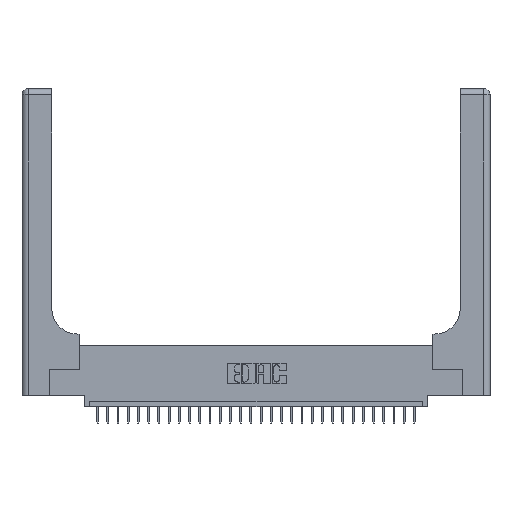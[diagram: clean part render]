
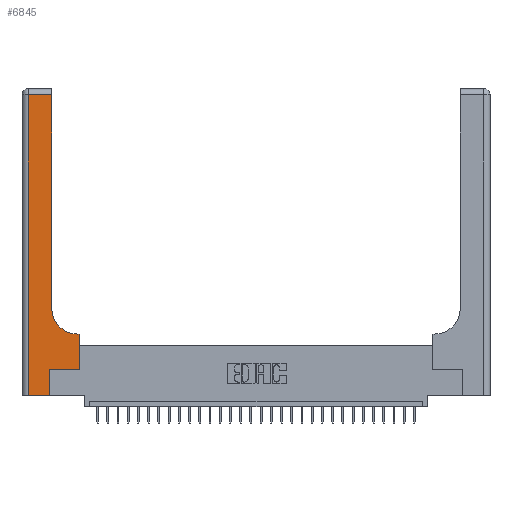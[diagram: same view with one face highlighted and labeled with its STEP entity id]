
A CAD part, top view. The second image highlights one B-rep face of the part: STEP entity #6845.
In plain terms, the highlighted planar face has unit normal (0, 0, 1).
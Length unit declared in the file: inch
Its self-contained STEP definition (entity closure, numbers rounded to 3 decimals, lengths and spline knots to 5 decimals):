
#518 = LINE ( 'NONE', #16669, #18775 ) ;
#1327 = EDGE_CURVE ( 'NONE', #23200, #5818, #17665, .T. ) ;
#1470 = LINE ( 'NONE', #10224, #26802 ) ;
#1552 = EDGE_CURVE ( 'NONE', #7677, #23200, #518, .T. ) ;
#1557 = LINE ( 'NONE', #10333, #20223 ) ;
#1687 = ORIENTED_EDGE ( 'NONE', *, *, #12350, .T. ) ;
#1708 = LINE ( 'NONE', #12631, #3224 ) ;
#2526 = LINE ( 'NONE', #12492, #4786 ) ;
#3224 = VECTOR ( 'NONE', #29449, 39.37008 ) ;
#3350 = ORIENTED_EDGE ( 'NONE', *, *, #1327, .T. ) ;
#3388 = DIRECTION ( 'NONE',  ( 1., 0., 0. ) ) ;
#4222 = CARTESIAN_POINT ( 'NONE',  ( 0.269, 0.25, 0.37 ) ) ;
#4494 = EDGE_CURVE ( 'NONE', #10274, #17500, #1470, .T. ) ;
#4786 = VECTOR ( 'NONE', #29008, 39.37008 ) ;
#4972 = CARTESIAN_POINT ( 'NONE',  ( 0.06, 0., 0.37 ) ) ;
#5176 = CARTESIAN_POINT ( 'NONE',  ( 0., 3., 0.37 ) ) ;
#5198 = EDGE_CURVE ( 'NONE', #5818, #10274, #10402, .T. ) ;
#5818 = VERTEX_POINT ( 'NONE', #23641 ) ;
#6048 = AXIS2_PLACEMENT_3D ( 'NONE', #5176, #26195, #28772 ) ;
#6405 = EDGE_CURVE ( 'NONE', #17410, #16630, #1708, .T. ) ;
#6845 = ADVANCED_FACE ( 'NONE', ( #12890 ), #23618, .F. ) ;
#7677 = VERTEX_POINT ( 'NONE', #22383 ) ;
#7987 = LINE ( 'NONE', #21259, #21742 ) ;
#8482 = LINE ( 'NONE', #29399, #28921 ) ;
#8766 = EDGE_LOOP ( 'NONE', ( #29319, #23403, #18683, #26585, #25383, #1687, #9169, #15467, #3350 ) ) ;
#9169 = ORIENTED_EDGE ( 'NONE', *, *, #18579, .T. ) ;
#9742 = AXIS2_PLACEMENT_3D ( 'NONE', #12566, #19929, #3388 ) ;
#10224 = CARTESIAN_POINT ( 'NONE',  ( 0., 2.94, 0.37 ) ) ;
#10274 = VERTEX_POINT ( 'NONE', #20824 ) ;
#10333 = CARTESIAN_POINT ( 'NONE',  ( 0.269, 0., 0.37 ) ) ;
#10402 = LINE ( 'NONE', #13974, #25303 ) ;
#11852 = DIRECTION ( 'NONE',  ( 0., 1., 0. ) ) ;
#12192 = CARTESIAN_POINT ( 'NONE',  ( 0.5415, 0.6, 0.37 ) ) ;
#12350 = EDGE_CURVE ( 'NONE', #22232, #18464, #2526, .T. ) ;
#12492 = CARTESIAN_POINT ( 'NONE',  ( 0.269, 0.25, 0.37 ) ) ;
#12566 = CARTESIAN_POINT ( 'NONE',  ( 0.5415, 0.85, 0.37 ) ) ;
#12631 = CARTESIAN_POINT ( 'NONE',  ( 0., 0., 0.37 ) ) ;
#12683 = DIRECTION ( 'NONE',  ( 0., -1., 0. ) ) ;
#12890 = FACE_OUTER_BOUND ( 'NONE', #8766, .T. ) ;
#13974 = CARTESIAN_POINT ( 'NONE',  ( 0.2915, 3., 0.37 ) ) ;
#15290 = CARTESIAN_POINT ( 'NONE',  ( 0.269, 0., 0.37 ) ) ;
#15467 = ORIENTED_EDGE ( 'NONE', *, *, #1552, .T. ) ;
#16153 = DIRECTION ( 'NONE',  ( 0., 1., 0. ) ) ;
#16630 = VERTEX_POINT ( 'NONE', #15290 ) ;
#16669 = CARTESIAN_POINT ( 'NONE',  ( 0.2915, 0.6, 0.37 ) ) ;
#17410 = VERTEX_POINT ( 'NONE', #4972 ) ;
#17500 = VERTEX_POINT ( 'NONE', #22129 ) ;
#17665 = CIRCLE ( 'NONE', #9742, 0.25 ) ;
#18464 = VERTEX_POINT ( 'NONE', #28075 ) ;
#18579 = EDGE_CURVE ( 'NONE', #18464, #7677, #7987, .T. ) ;
#18683 = ORIENTED_EDGE ( 'NONE', *, *, #21689, .T. ) ;
#18775 = VECTOR ( 'NONE', #21479, 39.37008 ) ;
#19322 = EDGE_CURVE ( 'NONE', #16630, #22232, #1557, .T. ) ;
#19929 = DIRECTION ( 'NONE',  ( 0., 0., -1. ) ) ;
#20223 = VECTOR ( 'NONE', #21895, 39.37008 ) ;
#20824 = CARTESIAN_POINT ( 'NONE',  ( 0.2915, 2.94, 0.37 ) ) ;
#21259 = CARTESIAN_POINT ( 'NONE',  ( 0.5585, 0.25, 0.37 ) ) ;
#21479 = DIRECTION ( 'NONE',  ( -1., 0., 0. ) ) ;
#21689 = EDGE_CURVE ( 'NONE', #17500, #17410, #8482, .T. ) ;
#21742 = VECTOR ( 'NONE', #11852, 39.37008 ) ;
#21895 = DIRECTION ( 'NONE',  ( 0., 1., 0. ) ) ;
#22129 = CARTESIAN_POINT ( 'NONE',  ( 0.06, 2.94, 0.37 ) ) ;
#22232 = VERTEX_POINT ( 'NONE', #4222 ) ;
#22383 = CARTESIAN_POINT ( 'NONE',  ( 0.5585, 0.6, 0.37 ) ) ;
#23200 = VERTEX_POINT ( 'NONE', #12192 ) ;
#23403 = ORIENTED_EDGE ( 'NONE', *, *, #4494, .T. ) ;
#23618 = PLANE ( 'NONE',  #6048 ) ;
#23641 = CARTESIAN_POINT ( 'NONE',  ( 0.2915, 0.85, 0.37 ) ) ;
#25303 = VECTOR ( 'NONE', #16153, 39.37008 ) ;
#25383 = ORIENTED_EDGE ( 'NONE', *, *, #19322, .T. ) ;
#26195 = DIRECTION ( 'NONE',  ( 0., 0., -1. ) ) ;
#26585 = ORIENTED_EDGE ( 'NONE', *, *, #6405, .T. ) ;
#26802 = VECTOR ( 'NONE', #26956, 39.37008 ) ;
#26956 = DIRECTION ( 'NONE',  ( -1., 0., 0. ) ) ;
#28075 = CARTESIAN_POINT ( 'NONE',  ( 0.5585, 0.25, 0.37 ) ) ;
#28772 = DIRECTION ( 'NONE',  ( -1., 0., 0. ) ) ;
#28921 = VECTOR ( 'NONE', #12683, 39.37008 ) ;
#29008 = DIRECTION ( 'NONE',  ( 1., 0., 0. ) ) ;
#29319 = ORIENTED_EDGE ( 'NONE', *, *, #5198, .T. ) ;
#29399 = CARTESIAN_POINT ( 'NONE',  ( 0.06, 3., 0.37 ) ) ;
#29449 = DIRECTION ( 'NONE',  ( 1., 0., 0. ) ) ;
